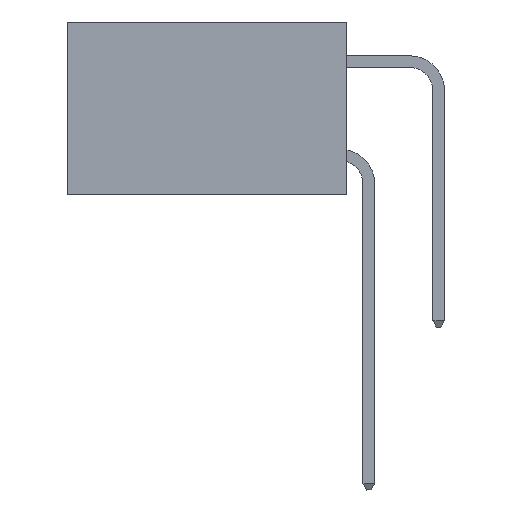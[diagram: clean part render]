
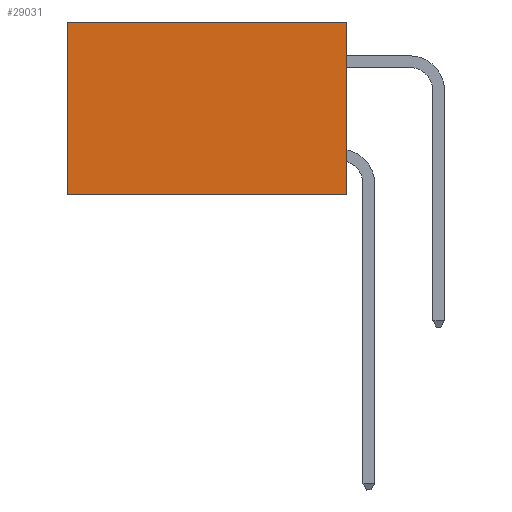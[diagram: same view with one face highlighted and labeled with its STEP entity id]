
A CAD part, left-side view. The second image highlights one B-rep face of the part: STEP entity #29031.
In plain terms, the highlighted planar face has unit normal (-1, 0, 0).
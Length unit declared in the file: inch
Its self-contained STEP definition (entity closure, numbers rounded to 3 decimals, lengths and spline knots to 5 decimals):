
#27 = CARTESIAN_POINT ( 'NONE',  ( 0.2875, 0., 0. ) ) ;
#2147 = CARTESIAN_POINT ( 'NONE',  ( 0.2875, 0.6, 0. ) ) ;
#2166 = CARTESIAN_POINT ( 'NONE',  ( 0.2875, 0., -0.37 ) ) ;
#2625 = LINE ( 'NONE', #24218, #40930 ) ;
#3580 = DIRECTION ( 'NONE',  ( 0., 1., 0. ) ) ;
#7921 = VERTEX_POINT ( 'NONE', #33376 ) ;
#8824 = CARTESIAN_POINT ( 'NONE',  ( 0.2875, 0.6, 0. ) ) ;
#9613 = FACE_OUTER_BOUND ( 'NONE', #15170, .T. ) ;
#9699 = ORIENTED_EDGE ( 'NONE', *, *, #38065, .F. ) ;
#13087 = AXIS2_PLACEMENT_3D ( 'NONE', #30421, #16837, #27255 ) ;
#13976 = ORIENTED_EDGE ( 'NONE', *, *, #17140, .T. ) ;
#15170 = EDGE_LOOP ( 'NONE', ( #13976, #38637, #9699, #31056 ) ) ;
#16837 = DIRECTION ( 'NONE',  ( 1., 0., 0. ) ) ;
#17140 = EDGE_CURVE ( 'NONE', #22830, #7921, #38274, .T. ) ;
#20290 = CARTESIAN_POINT ( 'NONE',  ( 0.2875, 0., 0. ) ) ;
#22027 = VECTOR ( 'NONE', #23259, 39.37008 ) ;
#22830 = VERTEX_POINT ( 'NONE', #8824 ) ;
#23259 = DIRECTION ( 'NONE',  ( 0., 1., 0. ) ) ;
#24218 = CARTESIAN_POINT ( 'NONE',  ( 0.2875, 0., 0. ) ) ;
#25141 = VECTOR ( 'NONE', #31126, 39.37008 ) ;
#26238 = LINE ( 'NONE', #20290, #25141 ) ;
#26920 = VECTOR ( 'NONE', #33336, 39.37008 ) ;
#27255 = DIRECTION ( 'NONE',  ( 0., 0., -1. ) ) ;
#28473 = EDGE_CURVE ( 'NONE', #43924, #7921, #31204, .T. ) ;
#28574 = VERTEX_POINT ( 'NONE', #27 ) ;
#29031 = ADVANCED_FACE ( 'NONE', ( #9613 ), #30998, .F. ) ;
#29079 = EDGE_CURVE ( 'NONE', #28574, #22830, #2625, .T. ) ;
#30421 = CARTESIAN_POINT ( 'NONE',  ( 0.2875, 0., 0. ) ) ;
#30998 = PLANE ( 'NONE',  #13087 ) ;
#31056 = ORIENTED_EDGE ( 'NONE', *, *, #29079, .T. ) ;
#31126 = DIRECTION ( 'NONE',  ( 0., 0., -1. ) ) ;
#31204 = LINE ( 'NONE', #2166, #22027 ) ;
#33336 = DIRECTION ( 'NONE',  ( 0., 0., -1. ) ) ;
#33376 = CARTESIAN_POINT ( 'NONE',  ( 0.2875, 0.6, -0.37 ) ) ;
#38065 = EDGE_CURVE ( 'NONE', #28574, #43924, #26238, .T. ) ;
#38274 = LINE ( 'NONE', #2147, #26920 ) ;
#38637 = ORIENTED_EDGE ( 'NONE', *, *, #28473, .F. ) ;
#40930 = VECTOR ( 'NONE', #3580, 39.37008 ) ;
#41309 = CARTESIAN_POINT ( 'NONE',  ( 0.2875, 0., -0.37 ) ) ;
#43924 = VERTEX_POINT ( 'NONE', #41309 ) ;
